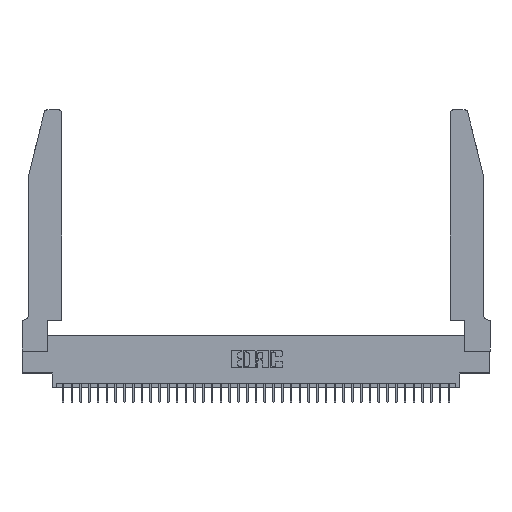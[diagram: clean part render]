
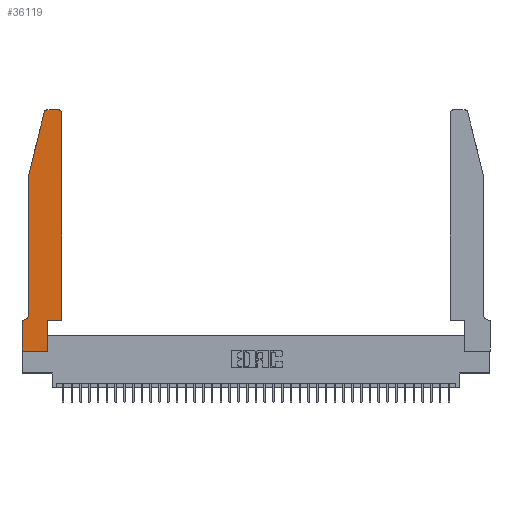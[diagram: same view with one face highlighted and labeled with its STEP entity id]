
A CAD part, top view. The second image highlights one B-rep face of the part: STEP entity #36119.
In plain terms, the highlighted planar face has unit normal (0, 0, 1).
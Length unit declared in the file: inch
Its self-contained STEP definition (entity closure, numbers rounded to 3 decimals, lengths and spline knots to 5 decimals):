
#88 = CARTESIAN_POINT ( 'NONE',  ( 0.0755, 0.42, 0.37 ) ) ;
#504 = VECTOR ( 'NONE', #23690, 39.37008 ) ;
#1178 = VERTEX_POINT ( 'NONE', #16813 ) ;
#1183 = AXIS2_PLACEMENT_3D ( 'NONE', #28800, #10430, #31877 ) ;
#1276 = VECTOR ( 'NONE', #18052, 39.37008 ) ;
#1332 = CARTESIAN_POINT ( 'NONE',  ( 0.4505, 0.35, 0.37 ) ) ;
#1606 = ORIENTED_EDGE ( 'NONE', *, *, #36454, .T. ) ;
#1699 = VERTEX_POINT ( 'NONE', #23622 ) ;
#1907 = EDGE_CURVE ( 'NONE', #29915, #24869, #2262, .T. ) ;
#2262 = LINE ( 'NONE', #33364, #1276 ) ;
#2426 = EDGE_CURVE ( 'NONE', #1178, #1699, #24959, .T. ) ;
#2440 = ORIENTED_EDGE ( 'NONE', *, *, #10018, .T. ) ;
#2472 = CARTESIAN_POINT ( 'NONE',  ( 0.2865, 0.35, 0.37 ) ) ;
#4169 = DIRECTION ( 'NONE',  ( 0., 0., 1. ) ) ;
#4214 = VERTEX_POINT ( 'NONE', #8207 ) ;
#4317 = EDGE_CURVE ( 'NONE', #27088, #6465, #13481, .T. ) ;
#5341 = CARTESIAN_POINT ( 'NONE',  ( 0.4205, 2.75, 0.37 ) ) ;
#5756 = ORIENTED_EDGE ( 'NONE', *, *, #4317, .T. ) ;
#6465 = VERTEX_POINT ( 'NONE', #19448 ) ;
#6594 = CARTESIAN_POINT ( 'NONE',  ( 0.284, 2.72, 0.37 ) ) ;
#7207 = EDGE_CURVE ( 'NONE', #22140, #29915, #17992, .T. ) ;
#8056 = ORIENTED_EDGE ( 'NONE', *, *, #7207, .T. ) ;
#8145 = EDGE_CURVE ( 'NONE', #1699, #22140, #24705, .T. ) ;
#8207 = CARTESIAN_POINT ( 'NONE',  ( 0.284, 2.75, 0.37 ) ) ;
#8908 = LINE ( 'NONE', #35868, #504 ) ;
#8979 = LINE ( 'NONE', #2472, #39584 ) ;
#9503 = DIRECTION ( 'NONE',  ( -1., 0., 0. ) ) ;
#9758 = DIRECTION ( 'NONE',  ( 1., 0., 0. ) ) ;
#10018 = EDGE_CURVE ( 'NONE', #28101, #28853, #12260, .T. ) ;
#10236 = DIRECTION ( 'NONE',  ( 0., -1., 0. ) ) ;
#10263 = ORIENTED_EDGE ( 'NONE', *, *, #2426, .T. ) ;
#10430 = DIRECTION ( 'NONE',  ( 0., 0., -1. ) ) ;
#11773 = DIRECTION ( 'NONE',  ( 0., 1., 0. ) ) ;
#12231 = CIRCLE ( 'NONE', #19312, 0.03 ) ;
#12260 = LINE ( 'NONE', #34907, #27593 ) ;
#12526 = VECTOR ( 'NONE', #27030, 39.37008 ) ;
#12986 = ORIENTED_EDGE ( 'NONE', *, *, #36046, .T. ) ;
#13145 = CARTESIAN_POINT ( 'NONE',  ( 0.4205, 2.72, 0.37 ) ) ;
#13466 = DIRECTION ( 'NONE',  ( 1., 0., 0. ) ) ;
#13481 = LINE ( 'NONE', #33193, #12526 ) ;
#13623 = VECTOR ( 'NONE', #9503, 39.37008 ) ;
#15062 = ORIENTED_EDGE ( 'NONE', *, *, #34688, .T. ) ;
#16218 = DIRECTION ( 'NONE',  ( 1., 0., 0. ) ) ;
#16493 = PLANE ( 'NONE',  #38763 ) ;
#16565 = VECTOR ( 'NONE', #38813, 39.37008 ) ;
#16813 = CARTESIAN_POINT ( 'NONE',  ( 0.25487, 2.72718, 0.37 ) ) ;
#17308 = CARTESIAN_POINT ( 'NONE',  ( 0.0755, 2., 0.37 ) ) ;
#17992 = CIRCLE ( 'NONE', #1183, 0.07 ) ;
#18052 = DIRECTION ( 'NONE',  ( -1., 0., 0. ) ) ;
#18616 = FACE_OUTER_BOUND ( 'NONE', #24885, .T. ) ;
#18622 = CARTESIAN_POINT ( 'NONE',  ( 0.2605, 2.75, 0.37 ) ) ;
#19312 = AXIS2_PLACEMENT_3D ( 'NONE', #6594, #28112, #9758 ) ;
#19448 = CARTESIAN_POINT ( 'NONE',  ( 0.2865, 0., 0.37 ) ) ;
#19651 = ORIENTED_EDGE ( 'NONE', *, *, #8145, .T. ) ;
#20852 = CARTESIAN_POINT ( 'NONE',  ( 0.0755, 2., 0.37 ) ) ;
#21288 = VECTOR ( 'NONE', #10236, 39.37008 ) ;
#21858 = CARTESIAN_POINT ( 'NONE',  ( 0.0055, 0.35, 0.37 ) ) ;
#22140 = VERTEX_POINT ( 'NONE', #88 ) ;
#22644 = CARTESIAN_POINT ( 'NONE',  ( 0., 0.35, 0.37 ) ) ;
#22799 = EDGE_CURVE ( 'NONE', #36991, #4214, #29916, .T. ) ;
#23622 = CARTESIAN_POINT ( 'NONE',  ( 0.0755, 2., 0.37 ) ) ;
#23690 = DIRECTION ( 'NONE',  ( 0., 1., 0. ) ) ;
#24277 = ORIENTED_EDGE ( 'NONE', *, *, #39438, .T. ) ;
#24383 = ORIENTED_EDGE ( 'NONE', *, *, #27756, .T. ) ;
#24468 = AXIS2_PLACEMENT_3D ( 'NONE', #13145, #34594, #16218 ) ;
#24705 = LINE ( 'NONE', #17308, #16565 ) ;
#24869 = VERTEX_POINT ( 'NONE', #34297 ) ;
#24885 = EDGE_LOOP ( 'NONE', ( #33810, #15062, #10263, #19651, #8056, #39149, #24277, #5756, #1606, #2440, #24383, #12986 ) ) ;
#24959 = LINE ( 'NONE', #20852, #39249 ) ;
#25748 = DIRECTION ( 'NONE',  ( 1., 0., 0. ) ) ;
#26804 = VERTEX_POINT ( 'NONE', #34909 ) ;
#27030 = DIRECTION ( 'NONE',  ( 1., 0., 0. ) ) ;
#27088 = VERTEX_POINT ( 'NONE', #33020 ) ;
#27593 = VECTOR ( 'NONE', #13466, 39.37008 ) ;
#27756 = EDGE_CURVE ( 'NONE', #28853, #26804, #8908, .T. ) ;
#28101 = VERTEX_POINT ( 'NONE', #34544 ) ;
#28112 = DIRECTION ( 'NONE',  ( 0., 0., 1. ) ) ;
#28800 = CARTESIAN_POINT ( 'NONE',  ( 0.0055, 0.42, 0.37 ) ) ;
#28853 = VERTEX_POINT ( 'NONE', #1332 ) ;
#29915 = VERTEX_POINT ( 'NONE', #21858 ) ;
#29916 = LINE ( 'NONE', #18622, #13623 ) ;
#31601 = CIRCLE ( 'NONE', #24468, 0.03 ) ;
#31694 = CARTESIAN_POINT ( 'NONE',  ( 0., 0., 0.37 ) ) ;
#31877 = DIRECTION ( 'NONE',  ( -1., 0., 0. ) ) ;
#33020 = CARTESIAN_POINT ( 'NONE',  ( 0., 0., 0.37 ) ) ;
#33057 = DIRECTION ( 'NONE',  ( -0.239, -0.971, 0. ) ) ;
#33193 = CARTESIAN_POINT ( 'NONE',  ( 0., 0., 0.37 ) ) ;
#33364 = CARTESIAN_POINT ( 'NONE',  ( 0.0755, 0.35, 0.37 ) ) ;
#33810 = ORIENTED_EDGE ( 'NONE', *, *, #22799, .T. ) ;
#34297 = CARTESIAN_POINT ( 'NONE',  ( 0., 0.35, 0.37 ) ) ;
#34544 = CARTESIAN_POINT ( 'NONE',  ( 0.2865, 0.35, 0.37 ) ) ;
#34594 = DIRECTION ( 'NONE',  ( 0., 0., 1. ) ) ;
#34688 = EDGE_CURVE ( 'NONE', #4214, #1178, #12231, .T. ) ;
#34907 = CARTESIAN_POINT ( 'NONE',  ( 0.4505, 0.35, 0.37 ) ) ;
#34909 = CARTESIAN_POINT ( 'NONE',  ( 0.4505, 2.72, 0.37 ) ) ;
#35868 = CARTESIAN_POINT ( 'NONE',  ( 0.4505, 0.35, 0.37 ) ) ;
#36046 = EDGE_CURVE ( 'NONE', #26804, #36991, #31601, .T. ) ;
#36119 = ADVANCED_FACE ( 'NONE', ( #18616 ), #16493, .T. ) ;
#36454 = EDGE_CURVE ( 'NONE', #6465, #28101, #8979, .T. ) ;
#36589 = LINE ( 'NONE', #31694, #21288 ) ;
#36991 = VERTEX_POINT ( 'NONE', #5341 ) ;
#38763 = AXIS2_PLACEMENT_3D ( 'NONE', #22644, #4169, #25748 ) ;
#38813 = DIRECTION ( 'NONE',  ( 0., -1., 0. ) ) ;
#39149 = ORIENTED_EDGE ( 'NONE', *, *, #1907, .T. ) ;
#39249 = VECTOR ( 'NONE', #33057, 39.37008 ) ;
#39438 = EDGE_CURVE ( 'NONE', #24869, #27088, #36589, .T. ) ;
#39584 = VECTOR ( 'NONE', #11773, 39.37008 ) ;
